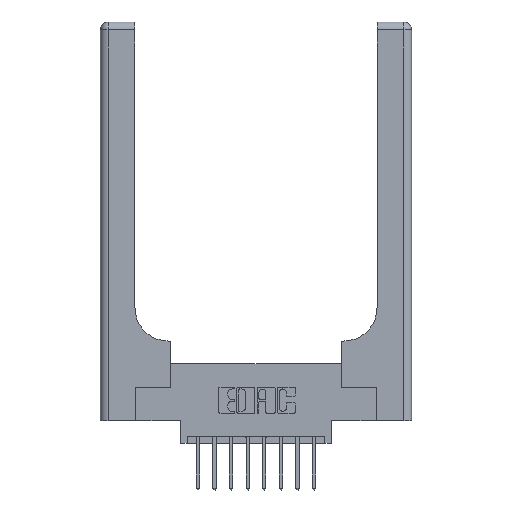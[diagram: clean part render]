
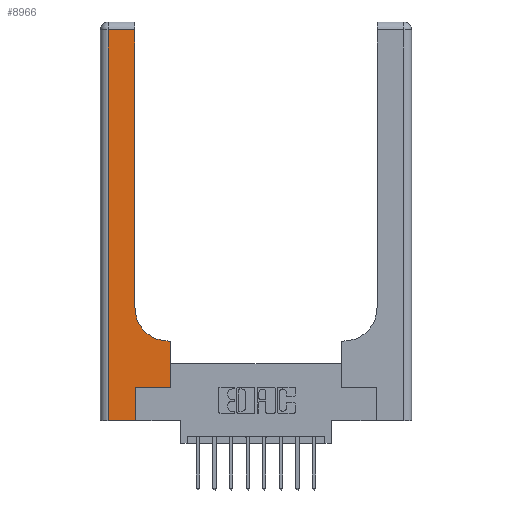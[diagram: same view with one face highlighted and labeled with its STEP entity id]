
A CAD part, top view. The second image highlights one B-rep face of the part: STEP entity #8966.
In plain terms, the highlighted planar face has unit normal (0, 0, 1).
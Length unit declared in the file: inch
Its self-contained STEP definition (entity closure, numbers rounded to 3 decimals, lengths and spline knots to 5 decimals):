
#249 = VECTOR ( 'NONE', #6747, 39.37008 ) ;
#582 = ORIENTED_EDGE ( 'NONE', *, *, #9540, .T. ) ;
#626 = DIRECTION ( 'NONE',  ( 0., 0., -1. ) ) ;
#666 = EDGE_CURVE ( 'NONE', #998, #4192, #5073, .T. ) ;
#998 = VERTEX_POINT ( 'NONE', #10553 ) ;
#1421 = CARTESIAN_POINT ( 'NONE',  ( 0.26, 2.94, 0.37 ) ) ;
#1457 = VERTEX_POINT ( 'NONE', #4229 ) ;
#1579 = VECTOR ( 'NONE', #2478, 39.37008 ) ;
#1620 = EDGE_CURVE ( 'NONE', #4066, #13053, #7810, .T. ) ;
#1764 = DIRECTION ( 'NONE',  ( 0., 1., 0. ) ) ;
#1972 = VECTOR ( 'NONE', #13525, 39.37008 ) ;
#2031 = VECTOR ( 'NONE', #14639, 39.37008 ) ;
#2086 = CARTESIAN_POINT ( 'NONE',  ( 0.06, 3., 0.37 ) ) ;
#2303 = EDGE_CURVE ( 'NONE', #13053, #1457, #11440, .T. ) ;
#2478 = DIRECTION ( 'NONE',  ( -1., 0., 0. ) ) ;
#2865 = CARTESIAN_POINT ( 'NONE',  ( 0.26, 0.6, 0.37 ) ) ;
#3174 = EDGE_CURVE ( 'NONE', #13835, #998, #4280, .T. ) ;
#3293 = CARTESIAN_POINT ( 'NONE',  ( 0.265, 0., 0.37 ) ) ;
#4066 = VERTEX_POINT ( 'NONE', #13260 ) ;
#4079 = LINE ( 'NONE', #9948, #4440 ) ;
#4192 = VERTEX_POINT ( 'NONE', #13808 ) ;
#4229 = CARTESIAN_POINT ( 'NONE',  ( 0.26, 0.85, 0.37 ) ) ;
#4280 = LINE ( 'NONE', #2086, #13606 ) ;
#4355 = ORIENTED_EDGE ( 'NONE', *, *, #5658, .T. ) ;
#4440 = VECTOR ( 'NONE', #1764, 39.37008 ) ;
#4541 = LINE ( 'NONE', #11357, #10400 ) ;
#4826 = EDGE_CURVE ( 'NONE', #10417, #13835, #11007, .T. ) ;
#5073 = LINE ( 'NONE', #13652, #1972 ) ;
#5286 = FACE_OUTER_BOUND ( 'NONE', #12458, .T. ) ;
#5658 = EDGE_CURVE ( 'NONE', #4192, #9493, #6480, .T. ) ;
#5885 = CARTESIAN_POINT ( 'NONE',  ( 0.51, 0.85, 0.37 ) ) ;
#6118 = EDGE_CURVE ( 'NONE', #12160, #4066, #4079, .T. ) ;
#6480 = LINE ( 'NONE', #3293, #249 ) ;
#6747 = DIRECTION ( 'NONE',  ( 0., 1., 0. ) ) ;
#7079 = DIRECTION ( 'NONE',  ( 1., 0., 0. ) ) ;
#7231 = ORIENTED_EDGE ( 'NONE', *, *, #666, .T. ) ;
#7309 = AXIS2_PLACEMENT_3D ( 'NONE', #5885, #14073, #7079 ) ;
#7639 = CARTESIAN_POINT ( 'NONE',  ( 0., 2.94, 0.37 ) ) ;
#7642 = CARTESIAN_POINT ( 'NONE',  ( 0., 3., 0.37 ) ) ;
#7810 = LINE ( 'NONE', #2865, #1579 ) ;
#8417 = CARTESIAN_POINT ( 'NONE',  ( 0.51, 0.6, 0.37 ) ) ;
#8634 = ORIENTED_EDGE ( 'NONE', *, *, #1620, .T. ) ;
#8830 = DIRECTION ( 'NONE',  ( -1., 0., 0. ) ) ;
#8966 = ADVANCED_FACE ( 'NONE', ( #5286 ), #9934, .F. ) ;
#9078 = LINE ( 'NONE', #9619, #12176 ) ;
#9493 = VERTEX_POINT ( 'NONE', #10122 ) ;
#9540 = EDGE_CURVE ( 'NONE', #1457, #10417, #4541, .T. ) ;
#9619 = CARTESIAN_POINT ( 'NONE',  ( 0.265, 0.25, 0.37 ) ) ;
#9934 = PLANE ( 'NONE',  #14309 ) ;
#9948 = CARTESIAN_POINT ( 'NONE',  ( 0.528, 0.25, 0.37 ) ) ;
#9959 = CARTESIAN_POINT ( 'NONE',  ( 0.06, 2.94, 0.37 ) ) ;
#10122 = CARTESIAN_POINT ( 'NONE',  ( 0.265, 0.25, 0.37 ) ) ;
#10400 = VECTOR ( 'NONE', #14878, 39.37008 ) ;
#10417 = VERTEX_POINT ( 'NONE', #1421 ) ;
#10553 = CARTESIAN_POINT ( 'NONE',  ( 0.06, 0., 0.37 ) ) ;
#10864 = ORIENTED_EDGE ( 'NONE', *, *, #6118, .T. ) ;
#11007 = LINE ( 'NONE', #7639, #2031 ) ;
#11357 = CARTESIAN_POINT ( 'NONE',  ( 0.26, 3., 0.37 ) ) ;
#11440 = CIRCLE ( 'NONE', #7309, 0.25 ) ;
#11443 = DIRECTION ( 'NONE',  ( 0., -1., 0. ) ) ;
#11537 = EDGE_CURVE ( 'NONE', #9493, #12160, #9078, .T. ) ;
#12160 = VERTEX_POINT ( 'NONE', #13136 ) ;
#12172 = ORIENTED_EDGE ( 'NONE', *, *, #3174, .T. ) ;
#12176 = VECTOR ( 'NONE', #13154, 39.37008 ) ;
#12458 = EDGE_LOOP ( 'NONE', ( #582, #14919, #12172, #7231, #4355, #12948, #10864, #8634, #13520 ) ) ;
#12948 = ORIENTED_EDGE ( 'NONE', *, *, #11537, .T. ) ;
#13053 = VERTEX_POINT ( 'NONE', #8417 ) ;
#13136 = CARTESIAN_POINT ( 'NONE',  ( 0.528, 0.25, 0.37 ) ) ;
#13154 = DIRECTION ( 'NONE',  ( 1., 0., 0. ) ) ;
#13260 = CARTESIAN_POINT ( 'NONE',  ( 0.528, 0.6, 0.37 ) ) ;
#13520 = ORIENTED_EDGE ( 'NONE', *, *, #2303, .T. ) ;
#13525 = DIRECTION ( 'NONE',  ( 1., 0., 0. ) ) ;
#13606 = VECTOR ( 'NONE', #11443, 39.37008 ) ;
#13652 = CARTESIAN_POINT ( 'NONE',  ( 0., 0., 0.37 ) ) ;
#13808 = CARTESIAN_POINT ( 'NONE',  ( 0.265, 0., 0.37 ) ) ;
#13835 = VERTEX_POINT ( 'NONE', #9959 ) ;
#14073 = DIRECTION ( 'NONE',  ( 0., 0., -1. ) ) ;
#14309 = AXIS2_PLACEMENT_3D ( 'NONE', #7642, #626, #8830 ) ;
#14639 = DIRECTION ( 'NONE',  ( -1., 0., 0. ) ) ;
#14878 = DIRECTION ( 'NONE',  ( 0., 1., 0. ) ) ;
#14919 = ORIENTED_EDGE ( 'NONE', *, *, #4826, .T. ) ;
